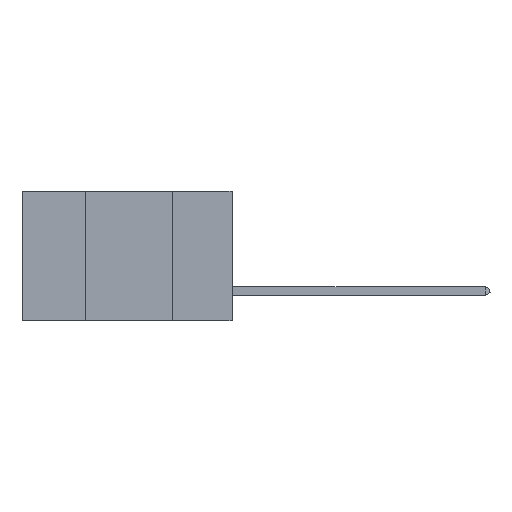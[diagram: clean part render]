
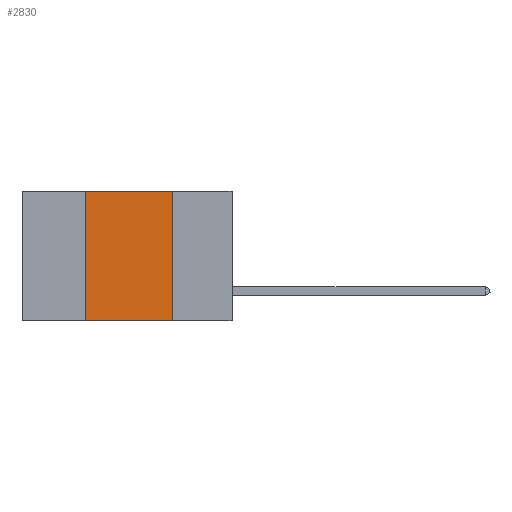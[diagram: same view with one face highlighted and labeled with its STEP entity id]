
A CAD part, left-side view. The second image highlights one B-rep face of the part: STEP entity #2830.
In plain terms, the highlighted planar face has unit normal (-1, 0, 0).
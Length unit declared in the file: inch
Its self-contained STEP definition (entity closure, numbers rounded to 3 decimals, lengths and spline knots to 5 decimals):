
#18 = VECTOR ( 'NONE', #5056, 39.37008 ) ;
#60 = CARTESIAN_POINT ( 'NONE',  ( 0., 0.42, 0. ) ) ;
#1566 = CARTESIAN_POINT ( 'NONE',  ( 0., 0.42, -0.37 ) ) ;
#1917 = DIRECTION ( 'NONE',  ( 1., 0., 0. ) ) ;
#2069 = VERTEX_POINT ( 'NONE', #4824 ) ;
#2263 = EDGE_CURVE ( 'NONE', #13660, #7340, #3092, .T. ) ;
#2676 = CARTESIAN_POINT ( 'NONE',  ( 0., 0.17, 0. ) ) ;
#2778 = CARTESIAN_POINT ( 'NONE',  ( 0., 0.6, -0.37 ) ) ;
#2814 = ORIENTED_EDGE ( 'NONE', *, *, #10811, .F. ) ;
#2830 = ADVANCED_FACE ( 'NONE', ( #8422 ), #11057, .F. ) ;
#2863 = ORIENTED_EDGE ( 'NONE', *, *, #13743, .F. ) ;
#3092 = LINE ( 'NONE', #14138, #18 ) ;
#4204 = VECTOR ( 'NONE', #7191, 39.37008 ) ;
#4824 = CARTESIAN_POINT ( 'NONE',  ( 0., 0.17, -0.37 ) ) ;
#5056 = DIRECTION ( 'NONE',  ( 0., 0., 1. ) ) ;
#5162 = VECTOR ( 'NONE', #10337, 39.37008 ) ;
#6899 = AXIS2_PLACEMENT_3D ( 'NONE', #14508, #1917, #9970 ) ;
#7191 = DIRECTION ( 'NONE',  ( 0., -1., 0. ) ) ;
#7340 = VERTEX_POINT ( 'NONE', #60 ) ;
#7561 = ORIENTED_EDGE ( 'NONE', *, *, #2263, .F. ) ;
#8027 = VERTEX_POINT ( 'NONE', #2676 ) ;
#8422 = FACE_OUTER_BOUND ( 'NONE', #9495, .T. ) ;
#8651 = LINE ( 'NONE', #9446, #9573 ) ;
#9446 = CARTESIAN_POINT ( 'NONE',  ( 0., 0.17, 0. ) ) ;
#9495 = EDGE_LOOP ( 'NONE', ( #2863, #2814, #7561, #12449 ) ) ;
#9573 = VECTOR ( 'NONE', #11790, 39.37008 ) ;
#9970 = DIRECTION ( 'NONE',  ( 0., 0., -1. ) ) ;
#10337 = DIRECTION ( 'NONE',  ( 0., -1., 0. ) ) ;
#10811 = EDGE_CURVE ( 'NONE', #7340, #8027, #13620, .T. ) ;
#11057 = PLANE ( 'NONE',  #6899 ) ;
#11790 = DIRECTION ( 'NONE',  ( 0., 0., -1. ) ) ;
#11859 = CARTESIAN_POINT ( 'NONE',  ( 0., 0.6, 0. ) ) ;
#12449 = ORIENTED_EDGE ( 'NONE', *, *, #13350, .T. ) ;
#13350 = EDGE_CURVE ( 'NONE', #13660, #2069, #14424, .T. ) ;
#13620 = LINE ( 'NONE', #11859, #5162 ) ;
#13660 = VERTEX_POINT ( 'NONE', #1566 ) ;
#13743 = EDGE_CURVE ( 'NONE', #8027, #2069, #8651, .T. ) ;
#14138 = CARTESIAN_POINT ( 'NONE',  ( 0., 0.42, 0. ) ) ;
#14424 = LINE ( 'NONE', #2778, #4204 ) ;
#14508 = CARTESIAN_POINT ( 'NONE',  ( 0., 0.6, 0. ) ) ;
